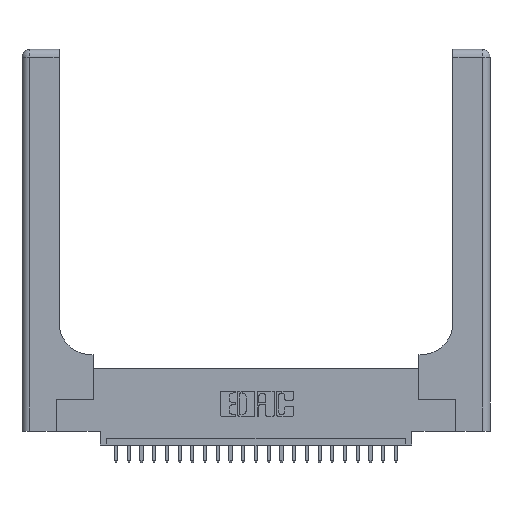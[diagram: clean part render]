
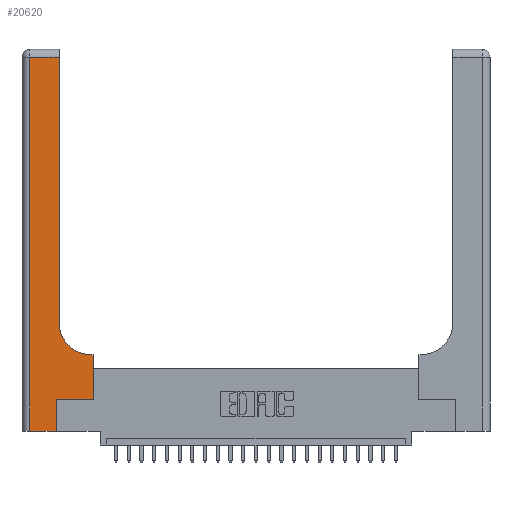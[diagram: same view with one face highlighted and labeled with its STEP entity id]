
A CAD part, top view. The second image highlights one B-rep face of the part: STEP entity #20620.
In plain terms, the highlighted planar face has unit normal (0, 0, 1).
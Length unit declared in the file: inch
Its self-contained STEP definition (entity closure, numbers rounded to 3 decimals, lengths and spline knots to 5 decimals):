
#184 = CARTESIAN_POINT ( 'NONE',  ( 0.269, 0.25, 0.37 ) ) ;
#345 = VERTEX_POINT ( 'NONE', #18080 ) ;
#638 = LINE ( 'NONE', #14140, #9069 ) ;
#873 = ORIENTED_EDGE ( 'NONE', *, *, #3024, .T. ) ;
#1075 = PLANE ( 'NONE',  #11302 ) ;
#1456 = DIRECTION ( 'NONE',  ( 1., 0., 0. ) ) ;
#2004 = EDGE_CURVE ( 'NONE', #20561, #6622, #18278, .T. ) ;
#2105 = VECTOR ( 'NONE', #7479, 39.37008 ) ;
#2890 = VERTEX_POINT ( 'NONE', #20459 ) ;
#3024 = EDGE_CURVE ( 'NONE', #2890, #20561, #16429, .T. ) ;
#3187 = VERTEX_POINT ( 'NONE', #21866 ) ;
#4182 = DIRECTION ( 'NONE',  ( 1., 0., 0. ) ) ;
#4261 = CARTESIAN_POINT ( 'NONE',  ( 0.06, 2.94, 0.37 ) ) ;
#4288 = ORIENTED_EDGE ( 'NONE', *, *, #11762, .T. ) ;
#4804 = ORIENTED_EDGE ( 'NONE', *, *, #2004, .T. ) ;
#4892 = EDGE_CURVE ( 'NONE', #6622, #7497, #7006, .T. ) ;
#4970 = DIRECTION ( 'NONE',  ( 0., 1., 0. ) ) ;
#5024 = DIRECTION ( 'NONE',  ( -1., 0., 0. ) ) ;
#5153 = LINE ( 'NONE', #12287, #9373 ) ;
#5603 = VECTOR ( 'NONE', #6287, 39.37008 ) ;
#6287 = DIRECTION ( 'NONE',  ( 0., 1., 0. ) ) ;
#6622 = VERTEX_POINT ( 'NONE', #16655 ) ;
#7006 = LINE ( 'NONE', #20716, #13991 ) ;
#7376 = DIRECTION ( 'NONE',  ( 0., 0., -1. ) ) ;
#7479 = DIRECTION ( 'NONE',  ( 0., 1., 0. ) ) ;
#7497 = VERTEX_POINT ( 'NONE', #4261 ) ;
#9027 = EDGE_LOOP ( 'NONE', ( #4804, #9185, #4288, #10097, #14602, #16245, #19355, #12119, #873 ) ) ;
#9057 = EDGE_CURVE ( 'NONE', #20603, #345, #19562, .T. ) ;
#9069 = VECTOR ( 'NONE', #14488, 39.37008 ) ;
#9185 = ORIENTED_EDGE ( 'NONE', *, *, #4892, .T. ) ;
#9276 = DIRECTION ( 'NONE',  ( 0., -1., 0. ) ) ;
#9373 = VECTOR ( 'NONE', #5024, 39.37008 ) ;
#10097 = ORIENTED_EDGE ( 'NONE', *, *, #23937, .T. ) ;
#10346 = CARTESIAN_POINT ( 'NONE',  ( 0.5585, 0.25, 0.37 ) ) ;
#10677 = CARTESIAN_POINT ( 'NONE',  ( 0.269, 0.25, 0.37 ) ) ;
#11302 = AXIS2_PLACEMENT_3D ( 'NONE', #19268, #7376, #24897 ) ;
#11335 = VERTEX_POINT ( 'NONE', #10677 ) ;
#11465 = CARTESIAN_POINT ( 'NONE',  ( 0.06, 3., 0.37 ) ) ;
#11762 = EDGE_CURVE ( 'NONE', #7497, #3187, #18106, .T. ) ;
#12119 = ORIENTED_EDGE ( 'NONE', *, *, #15835, .T. ) ;
#12287 = CARTESIAN_POINT ( 'NONE',  ( 0.2915, 0.6, 0.37 ) ) ;
#13070 = FACE_OUTER_BOUND ( 'NONE', #9027, .T. ) ;
#13991 = VECTOR ( 'NONE', #22352, 39.37008 ) ;
#14140 = CARTESIAN_POINT ( 'NONE',  ( 0., 0., 0.37 ) ) ;
#14488 = DIRECTION ( 'NONE',  ( 1., 0., 0. ) ) ;
#14574 = AXIS2_PLACEMENT_3D ( 'NONE', #24879, #16827, #1456 ) ;
#14602 = ORIENTED_EDGE ( 'NONE', *, *, #20837, .T. ) ;
#15835 = EDGE_CURVE ( 'NONE', #345, #2890, #5153, .T. ) ;
#15926 = CARTESIAN_POINT ( 'NONE',  ( 0.269, 0., 0.37 ) ) ;
#16097 = LINE ( 'NONE', #16148, #24351 ) ;
#16148 = CARTESIAN_POINT ( 'NONE',  ( 0.269, 0., 0.37 ) ) ;
#16245 = ORIENTED_EDGE ( 'NONE', *, *, #22474, .T. ) ;
#16429 = CIRCLE ( 'NONE', #14574, 0.25 ) ;
#16570 = VERTEX_POINT ( 'NONE', #15926 ) ;
#16655 = CARTESIAN_POINT ( 'NONE',  ( 0.2915, 2.94, 0.37 ) ) ;
#16827 = DIRECTION ( 'NONE',  ( 0., 0., -1. ) ) ;
#18080 = CARTESIAN_POINT ( 'NONE',  ( 0.5585, 0.6, 0.37 ) ) ;
#18106 = LINE ( 'NONE', #11465, #20240 ) ;
#18278 = LINE ( 'NONE', #24836, #2105 ) ;
#18803 = VECTOR ( 'NONE', #4182, 39.37008 ) ;
#19268 = CARTESIAN_POINT ( 'NONE',  ( 0., 3., 0.37 ) ) ;
#19355 = ORIENTED_EDGE ( 'NONE', *, *, #9057, .T. ) ;
#19385 = LINE ( 'NONE', #184, #18803 ) ;
#19562 = LINE ( 'NONE', #23719, #5603 ) ;
#20240 = VECTOR ( 'NONE', #9276, 39.37008 ) ;
#20459 = CARTESIAN_POINT ( 'NONE',  ( 0.5415, 0.6, 0.37 ) ) ;
#20561 = VERTEX_POINT ( 'NONE', #23260 ) ;
#20603 = VERTEX_POINT ( 'NONE', #10346 ) ;
#20620 = ADVANCED_FACE ( 'NONE', ( #13070 ), #1075, .F. ) ;
#20716 = CARTESIAN_POINT ( 'NONE',  ( 0., 2.94, 0.37 ) ) ;
#20837 = EDGE_CURVE ( 'NONE', #16570, #11335, #16097, .T. ) ;
#21866 = CARTESIAN_POINT ( 'NONE',  ( 0.06, 0., 0.37 ) ) ;
#22352 = DIRECTION ( 'NONE',  ( -1., 0., 0. ) ) ;
#22474 = EDGE_CURVE ( 'NONE', #11335, #20603, #19385, .T. ) ;
#23260 = CARTESIAN_POINT ( 'NONE',  ( 0.2915, 0.85, 0.37 ) ) ;
#23719 = CARTESIAN_POINT ( 'NONE',  ( 0.5585, 0.25, 0.37 ) ) ;
#23937 = EDGE_CURVE ( 'NONE', #3187, #16570, #638, .T. ) ;
#24351 = VECTOR ( 'NONE', #4970, 39.37008 ) ;
#24836 = CARTESIAN_POINT ( 'NONE',  ( 0.2915, 3., 0.37 ) ) ;
#24879 = CARTESIAN_POINT ( 'NONE',  ( 0.5415, 0.85, 0.37 ) ) ;
#24897 = DIRECTION ( 'NONE',  ( -1., 0., 0. ) ) ;
